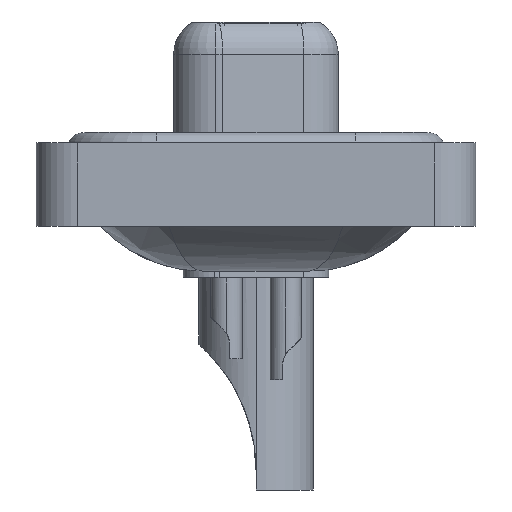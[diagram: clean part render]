
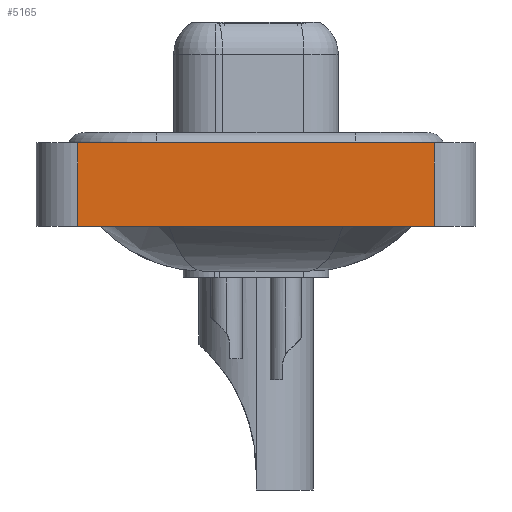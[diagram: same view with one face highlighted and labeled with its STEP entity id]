
A CAD part, left-side view. The second image highlights one B-rep face of the part: STEP entity #5165.
In plain terms, the highlighted planar face has unit normal (-1, 0, 0).
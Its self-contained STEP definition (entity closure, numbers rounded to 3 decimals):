
#521 = DIRECTION ( 'NONE',  ( -1., 0., 0. ) ) ;
#1751 = VERTEX_POINT ( 'NONE', #4385 ) ;
#2486 = EDGE_CURVE ( 'NONE', #8949, #12291, #8673, .T. ) ;
#3352 = VERTEX_POINT ( 'NONE', #19853 ) ;
#3424 = ORIENTED_EDGE ( 'NONE', *, *, #12282, .T. ) ;
#3714 = VECTOR ( 'NONE', #11251, 1000. ) ;
#3963 = CARTESIAN_POINT ( 'NONE',  ( -7.25, -8.55, 0.4 ) ) ;
#4385 = CARTESIAN_POINT ( 'NONE',  ( -7.25, -8.55, 0.4 ) ) ;
#4670 = ORIENTED_EDGE ( 'NONE', *, *, #13950, .T. ) ;
#5165 = ADVANCED_FACE ( 'NONE', ( #15792 ), #8145, .T. ) ;
#7141 = EDGE_LOOP ( 'NONE', ( #3424, #10212, #10719, #4670 ) ) ;
#7441 = CARTESIAN_POINT ( 'NONE',  ( -7.25, 8.55, -3.6 ) ) ;
#8033 = CARTESIAN_POINT ( 'NONE',  ( -7.25, -8.55, -3.6 ) ) ;
#8145 = PLANE ( 'NONE',  #11510 ) ;
#8238 = LINE ( 'NONE', #8033, #10756 ) ;
#8323 = LINE ( 'NONE', #19079, #3714 ) ;
#8388 = DIRECTION ( 'NONE',  ( 0., -1., 0. ) ) ;
#8673 = LINE ( 'NONE', #7441, #14782 ) ;
#8949 = VERTEX_POINT ( 'NONE', #14445 ) ;
#10212 = ORIENTED_EDGE ( 'NONE', *, *, #11351, .F. ) ;
#10712 = VECTOR ( 'NONE', #8388, 1000. ) ;
#10719 = ORIENTED_EDGE ( 'NONE', *, *, #2486, .F. ) ;
#10756 = VECTOR ( 'NONE', #14378, 1000. ) ;
#11251 = DIRECTION ( 'NONE',  ( 0., -1., 0. ) ) ;
#11351 = EDGE_CURVE ( 'NONE', #12291, #1751, #16039, .T. ) ;
#11510 = AXIS2_PLACEMENT_3D ( 'NONE', #14284, #521, #15238 ) ;
#12282 = EDGE_CURVE ( 'NONE', #3352, #1751, #8238, .T. ) ;
#12291 = VERTEX_POINT ( 'NONE', #12689 ) ;
#12689 = CARTESIAN_POINT ( 'NONE',  ( -7.25, 8.55, 0.4 ) ) ;
#13592 = DIRECTION ( 'NONE',  ( 0., 0., 1. ) ) ;
#13950 = EDGE_CURVE ( 'NONE', #8949, #3352, #8323, .T. ) ;
#14284 = CARTESIAN_POINT ( 'NONE',  ( -7.25, -8.55, -3.6 ) ) ;
#14378 = DIRECTION ( 'NONE',  ( 0., 0., 1. ) ) ;
#14445 = CARTESIAN_POINT ( 'NONE',  ( -7.25, 8.55, -3.6 ) ) ;
#14782 = VECTOR ( 'NONE', #13592, 1000. ) ;
#15238 = DIRECTION ( 'NONE',  ( 0., 0., 1. ) ) ;
#15792 = FACE_OUTER_BOUND ( 'NONE', #7141, .T. ) ;
#16039 = LINE ( 'NONE', #3963, #10712 ) ;
#19079 = CARTESIAN_POINT ( 'NONE',  ( -7.25, -8.55, -3.6 ) ) ;
#19853 = CARTESIAN_POINT ( 'NONE',  ( -7.25, -8.55, -3.6 ) ) ;
